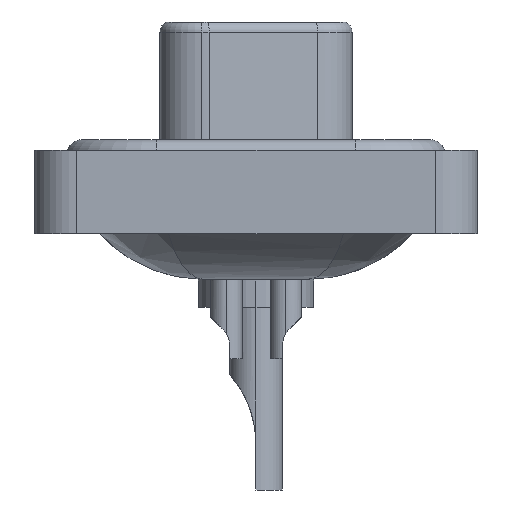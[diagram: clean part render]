
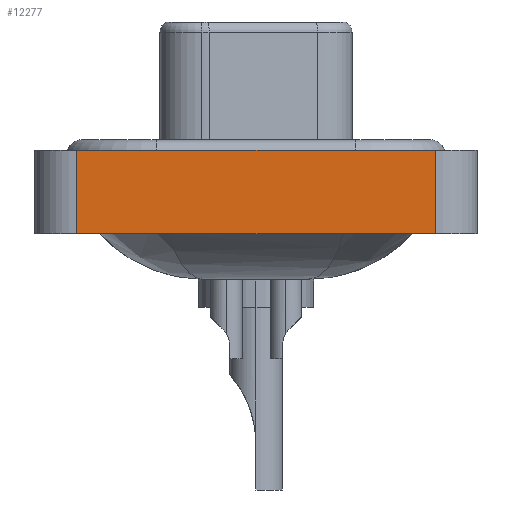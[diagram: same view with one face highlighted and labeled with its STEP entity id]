
A CAD part, left-side view. The second image highlights one B-rep face of the part: STEP entity #12277.
In plain terms, the highlighted planar face has unit normal (-1, 0, 0).
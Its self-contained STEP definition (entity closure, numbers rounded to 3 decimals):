
#618 = CARTESIAN_POINT ( 'NONE',  ( -7.25, -8.55, 0.4 ) ) ;
#1684 = ORIENTED_EDGE ( 'NONE', *, *, #9571, .T. ) ;
#2430 = VERTEX_POINT ( 'NONE', #618 ) ;
#2798 = LINE ( 'NONE', #17679, #15117 ) ;
#2979 = ORIENTED_EDGE ( 'NONE', *, *, #4584, .T. ) ;
#3091 = DIRECTION ( 'NONE',  ( 0., 0., 1. ) ) ;
#3116 = VERTEX_POINT ( 'NONE', #6832 ) ;
#4264 = PLANE ( 'NONE',  #5316 ) ;
#4424 = DIRECTION ( 'NONE',  ( 0., -1., 0. ) ) ;
#4544 = EDGE_CURVE ( 'NONE', #3116, #2430, #2798, .T. ) ;
#4584 = EDGE_CURVE ( 'NONE', #8737, #9400, #10973, .T. ) ;
#4695 = DIRECTION ( 'NONE',  ( 0., 0., 1. ) ) ;
#4837 = ORIENTED_EDGE ( 'NONE', *, *, #15993, .F. ) ;
#5316 = AXIS2_PLACEMENT_3D ( 'NONE', #5807, #14092, #3091 ) ;
#5399 = CARTESIAN_POINT ( 'NONE',  ( -7.25, 8.55, -3.6 ) ) ;
#5807 = CARTESIAN_POINT ( 'NONE',  ( -7.25, -8.55, -3.6 ) ) ;
#6063 = CARTESIAN_POINT ( 'NONE',  ( -7.25, 8.55, -3.6 ) ) ;
#6832 = CARTESIAN_POINT ( 'NONE',  ( -7.25, 8.55, 0.4 ) ) ;
#8345 = DIRECTION ( 'NONE',  ( 0., -1., 0. ) ) ;
#8617 = LINE ( 'NONE', #11436, #10310 ) ;
#8651 = CARTESIAN_POINT ( 'NONE',  ( -7.25, -8.55, -3.6 ) ) ;
#8737 = VERTEX_POINT ( 'NONE', #5399 ) ;
#8787 = DIRECTION ( 'NONE',  ( 0., 0., 1. ) ) ;
#9400 = VERTEX_POINT ( 'NONE', #8651 ) ;
#9456 = EDGE_LOOP ( 'NONE', ( #1684, #10134, #4837, #2979 ) ) ;
#9571 = EDGE_CURVE ( 'NONE', #9400, #2430, #8617, .T. ) ;
#10134 = ORIENTED_EDGE ( 'NONE', *, *, #4544, .F. ) ;
#10310 = VECTOR ( 'NONE', #8787, 1000. ) ;
#10973 = LINE ( 'NONE', #11606, #17157 ) ;
#11436 = CARTESIAN_POINT ( 'NONE',  ( -7.25, -8.55, -3.6 ) ) ;
#11606 = CARTESIAN_POINT ( 'NONE',  ( -7.25, -8.55, -3.6 ) ) ;
#11710 = LINE ( 'NONE', #6063, #17167 ) ;
#12277 = ADVANCED_FACE ( 'NONE', ( #16718 ), #4264, .T. ) ;
#14092 = DIRECTION ( 'NONE',  ( -1., 0., 0. ) ) ;
#15117 = VECTOR ( 'NONE', #8345, 1000. ) ;
#15993 = EDGE_CURVE ( 'NONE', #8737, #3116, #11710, .T. ) ;
#16718 = FACE_OUTER_BOUND ( 'NONE', #9456, .T. ) ;
#17157 = VECTOR ( 'NONE', #4424, 1000. ) ;
#17167 = VECTOR ( 'NONE', #4695, 1000. ) ;
#17679 = CARTESIAN_POINT ( 'NONE',  ( -7.25, -8.55, 0.4 ) ) ;
